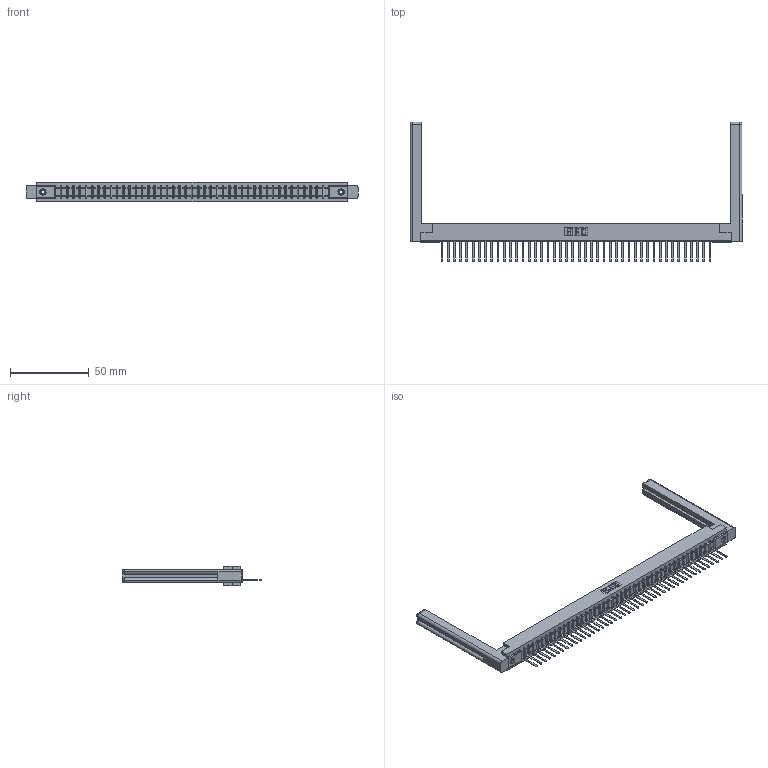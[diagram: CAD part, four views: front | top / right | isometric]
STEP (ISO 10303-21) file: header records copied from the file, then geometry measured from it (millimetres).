
FILE_DESCRIPTION (( 'STEP AP203' ), '1' );
FILE_NAME ('307-044-441-158.STEP', '2020-09-29T23:00:55', ( '' ), ( '' ), 'SwSTEP 2.0', 'SolidWorks 2020', '' );
FILE_SCHEMA (( 'CONFIG_CONTROL_DESIGN' ));
Length unit declared in the file: inch
Products named in the file (5): 307-290-002_541; 307-044-441-158; 307 Part_.156 Dia Mounting Holes; 345-250-001_345-250-001-102; 307-220-058
Assembly tree (49 placements, depth 2):
  307-044-441-158
    307 Part_.156 Dia Mounting Holes
    307-290-002_541  x44
    307-220-058  x2
    345-250-001_345-250-001-102  x2
Bounding box: 210.97 x 88.9 x 12.7 mm (x, y, z)
Volume: 29836 mm3; surface area: 34236.4 mm2
Topology: 49 solids, 49 shells, 3561 faces, 10885 edges, 7122 vertices
Faces by surface type: plane 2134, cylinder 1313, sphere 90, torus 12, cone 12
Entity records: 40825 total; most frequent: CARTESIAN_POINT 6895, ORIENTED_EDGE 6824, DIRECTION 6658, EDGE_CURVE 3412, VECTOR 2612, LINE 2612, VERTEX_POINT 2206, AXIS2_PLACEMENT_3D 2023
